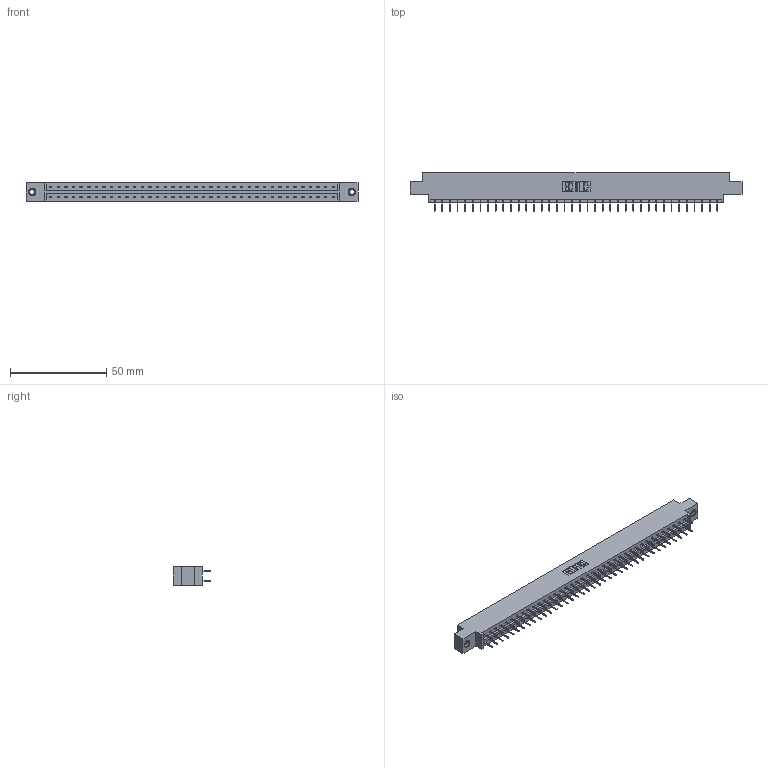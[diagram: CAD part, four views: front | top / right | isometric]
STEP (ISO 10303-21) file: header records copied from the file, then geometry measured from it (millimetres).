
FILE_DESCRIPTION (( 'STEP AP203' ), '1' );
FILE_NAME ('333-076-524-807.STEP', '2018-08-04T22:56:39', ( '' ), ( '' ), 'SwSTEP 2.0', 'SolidWorks 2016', '' );
FILE_SCHEMA (( 'CONFIG_CONTROL_DESIGN' ));
Length unit declared in the file: inch
Products named in the file (4): 333 Part_Offset - .156 Dia - TI; 345-292-001_345-293-124; 345-250-001_345-250-005-103; 333-076-524-807
Assembly tree (79 placements, depth 2):
  333-076-524-807
    333 Part_Offset - .156 Dia - TI
    345-292-001_345-293-124  x76
    345-250-001_345-250-005-103  x2
Bounding box: 172.11 x 19.69 x 9.4 mm (x, y, z)
Volume: 17177.8 mm3; surface area: 20175.2 mm2
Topology: 79 solids, 79 shells, 4434 faces, 12543 edges, 8050 vertices
Faces by surface type: plane 3298, cylinder 1120, cone 12, torus 4
Entity records: 26356 total; most frequent: CARTESIAN_POINT 4357, ORIENTED_EDGE 4286, DIRECTION 3761, EDGE_CURVE 2143, LINE 1999, VECTOR 1999, VERTEX_POINT 1420, AXIS2_PLACEMENT_3D 881
